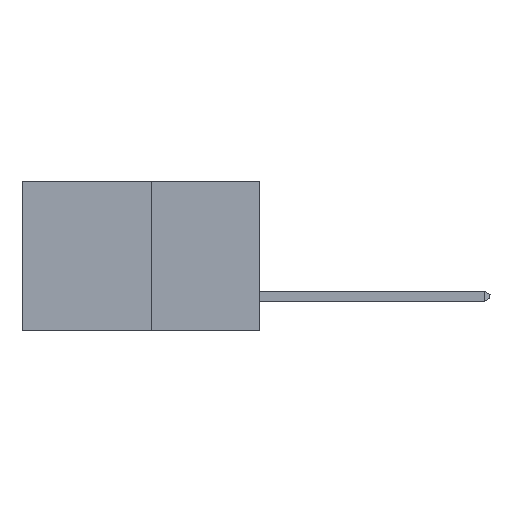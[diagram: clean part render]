
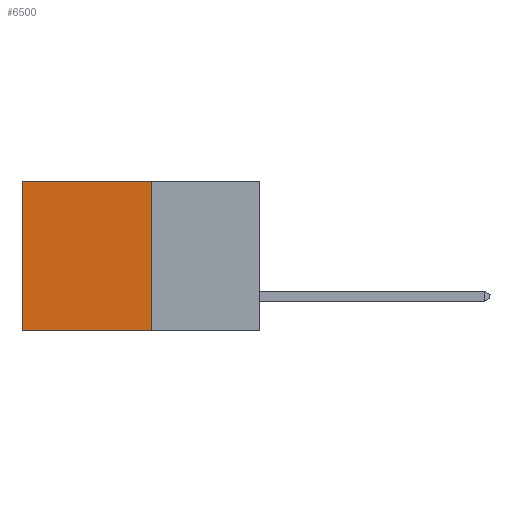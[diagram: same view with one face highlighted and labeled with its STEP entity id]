
A CAD part, left-side view. The second image highlights one B-rep face of the part: STEP entity #6500.
In plain terms, the highlighted planar face has unit normal (-1, 0, 0).
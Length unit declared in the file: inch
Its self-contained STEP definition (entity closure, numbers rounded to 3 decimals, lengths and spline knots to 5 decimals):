
#111 = CARTESIAN_POINT ( 'NONE',  ( 0.277, 0.27, -0.37 ) ) ;
#208 = ORIENTED_EDGE ( 'NONE', *, *, #2283, .F. ) ;
#565 = CARTESIAN_POINT ( 'NONE',  ( 0.277, 0.27, 0. ) ) ;
#2283 = EDGE_CURVE ( 'NONE', #2608, #10428, #9825, .T. ) ;
#2608 = VERTEX_POINT ( 'NONE', #565 ) ;
#2660 = EDGE_LOOP ( 'NONE', ( #10989, #8901, #208, #6339 ) ) ;
#3516 = DIRECTION ( 'NONE',  ( 0., 1., 0. ) ) ;
#3777 = DIRECTION ( 'NONE',  ( 0., 0., -1. ) ) ;
#3904 = PLANE ( 'NONE',  #10850 ) ;
#4114 = FACE_OUTER_BOUND ( 'NONE', #2660, .T. ) ;
#4317 = VERTEX_POINT ( 'NONE', #10085 ) ;
#4344 = VERTEX_POINT ( 'NONE', #11885 ) ;
#4912 = DIRECTION ( 'NONE',  ( 0., 0., -1. ) ) ;
#6339 = ORIENTED_EDGE ( 'NONE', *, *, #7275, .T. ) ;
#6500 = ADVANCED_FACE ( 'NONE', ( #4114 ), #3904, .F. ) ;
#6571 = VECTOR ( 'NONE', #8070, 39.37008 ) ;
#6652 = VECTOR ( 'NONE', #3516, 39.37008 ) ;
#6714 = CARTESIAN_POINT ( 'NONE',  ( 0.277, 0.59, -0.37 ) ) ;
#6983 = CARTESIAN_POINT ( 'NONE',  ( 0.277, 0.27, 0. ) ) ;
#7275 = EDGE_CURVE ( 'NONE', #2608, #4317, #10110, .T. ) ;
#7385 = CARTESIAN_POINT ( 'NONE',  ( 0.277, 0.27, -0.37 ) ) ;
#7705 = EDGE_CURVE ( 'NONE', #4317, #4344, #12170, .T. ) ;
#7713 = VECTOR ( 'NONE', #9684, 39.37008 ) ;
#8070 = DIRECTION ( 'NONE',  ( 0., 0., -1. ) ) ;
#8177 = EDGE_CURVE ( 'NONE', #10428, #4344, #9064, .T. ) ;
#8260 = CARTESIAN_POINT ( 'NONE',  ( 0.277, 0.27, -0.37 ) ) ;
#8901 = ORIENTED_EDGE ( 'NONE', *, *, #8177, .F. ) ;
#9064 = LINE ( 'NONE', #7385, #6652 ) ;
#9684 = DIRECTION ( 'NONE',  ( 0., 1., 0. ) ) ;
#9825 = LINE ( 'NONE', #8260, #6571 ) ;
#10085 = CARTESIAN_POINT ( 'NONE',  ( 0.277, 0.59, 0. ) ) ;
#10110 = LINE ( 'NONE', #6983, #7713 ) ;
#10428 = VERTEX_POINT ( 'NONE', #111 ) ;
#10434 = DIRECTION ( 'NONE',  ( 1., 0., 0. ) ) ;
#10850 = AXIS2_PLACEMENT_3D ( 'NONE', #11289, #10434, #4912 ) ;
#10989 = ORIENTED_EDGE ( 'NONE', *, *, #7705, .T. ) ;
#11289 = CARTESIAN_POINT ( 'NONE',  ( 0.277, 0.27, -0.37 ) ) ;
#11883 = VECTOR ( 'NONE', #3777, 39.37008 ) ;
#11885 = CARTESIAN_POINT ( 'NONE',  ( 0.277, 0.59, -0.37 ) ) ;
#12170 = LINE ( 'NONE', #6714, #11883 ) ;
